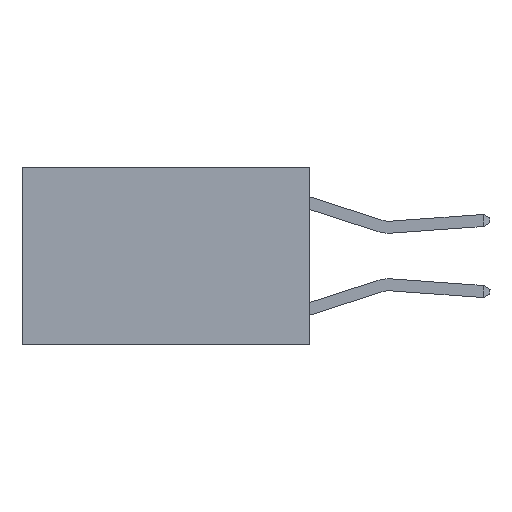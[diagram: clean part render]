
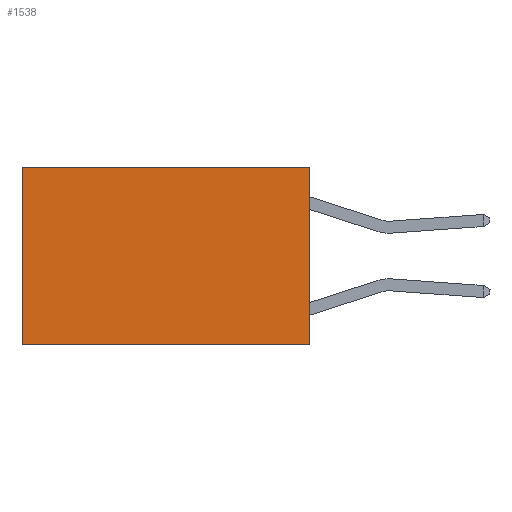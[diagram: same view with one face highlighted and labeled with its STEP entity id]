
A CAD part, left-side view. The second image highlights one B-rep face of the part: STEP entity #1538.
In plain terms, the highlighted planar face has unit normal (-1, 0, 0).
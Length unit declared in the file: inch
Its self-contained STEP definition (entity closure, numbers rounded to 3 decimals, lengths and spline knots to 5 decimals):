
#430 = CARTESIAN_POINT ( 'NONE',  ( 0.2625, 0., 0. ) ) ;
#1318 = EDGE_CURVE ( 'NONE', #7170, #10318, #7465, .T. ) ;
#1353 = DIRECTION ( 'NONE',  ( 0., 1., 0. ) ) ;
#1538 = ADVANCED_FACE ( 'NONE', ( #16571 ), #5748, .F. ) ;
#2086 = CARTESIAN_POINT ( 'NONE',  ( 0.2625, 0., 0. ) ) ;
#2271 = LINE ( 'NONE', #2086, #15597 ) ;
#2762 = VECTOR ( 'NONE', #11090, 39.37008 ) ;
#2888 = EDGE_CURVE ( 'NONE', #21374, #7170, #2271, .T. ) ;
#3353 = CARTESIAN_POINT ( 'NONE',  ( 0.2625, 0.6, 0. ) ) ;
#4064 = DIRECTION ( 'NONE',  ( 0., 0., -1. ) ) ;
#4484 = AXIS2_PLACEMENT_3D ( 'NONE', #14979, #13192, #4064 ) ;
#4706 = ORIENTED_EDGE ( 'NONE', *, *, #11670, .F. ) ;
#5384 = DIRECTION ( 'NONE',  ( 0., 1., 0. ) ) ;
#5748 = PLANE ( 'NONE',  #4484 ) ;
#5973 = CARTESIAN_POINT ( 'NONE',  ( 0.2625, 0.6, 0. ) ) ;
#6139 = CARTESIAN_POINT ( 'NONE',  ( 0.2625, 0., -0.37 ) ) ;
#7170 = VERTEX_POINT ( 'NONE', #5973 ) ;
#7245 = LINE ( 'NONE', #7734, #2762 ) ;
#7331 = EDGE_CURVE ( 'NONE', #19979, #10318, #8931, .T. ) ;
#7465 = LINE ( 'NONE', #3353, #21193 ) ;
#7734 = CARTESIAN_POINT ( 'NONE',  ( 0.2625, 0., 0. ) ) ;
#8416 = VECTOR ( 'NONE', #1353, 39.37008 ) ;
#8931 = LINE ( 'NONE', #11394, #8416 ) ;
#9090 = ORIENTED_EDGE ( 'NONE', *, *, #2888, .T. ) ;
#10318 = VERTEX_POINT ( 'NONE', #18769 ) ;
#10573 = DIRECTION ( 'NONE',  ( 0., 0., -1. ) ) ;
#11090 = DIRECTION ( 'NONE',  ( 0., 0., -1. ) ) ;
#11394 = CARTESIAN_POINT ( 'NONE',  ( 0.2625, 0., -0.37 ) ) ;
#11395 = EDGE_LOOP ( 'NONE', ( #14725, #14410, #4706, #9090 ) ) ;
#11670 = EDGE_CURVE ( 'NONE', #21374, #19979, #7245, .T. ) ;
#13192 = DIRECTION ( 'NONE',  ( 1., 0., 0. ) ) ;
#14410 = ORIENTED_EDGE ( 'NONE', *, *, #7331, .F. ) ;
#14725 = ORIENTED_EDGE ( 'NONE', *, *, #1318, .T. ) ;
#14979 = CARTESIAN_POINT ( 'NONE',  ( 0.2625, 0., 0. ) ) ;
#15597 = VECTOR ( 'NONE', #5384, 39.37008 ) ;
#16571 = FACE_OUTER_BOUND ( 'NONE', #11395, .T. ) ;
#18769 = CARTESIAN_POINT ( 'NONE',  ( 0.2625, 0.6, -0.37 ) ) ;
#19979 = VERTEX_POINT ( 'NONE', #6139 ) ;
#21193 = VECTOR ( 'NONE', #10573, 39.37008 ) ;
#21374 = VERTEX_POINT ( 'NONE', #430 ) ;
